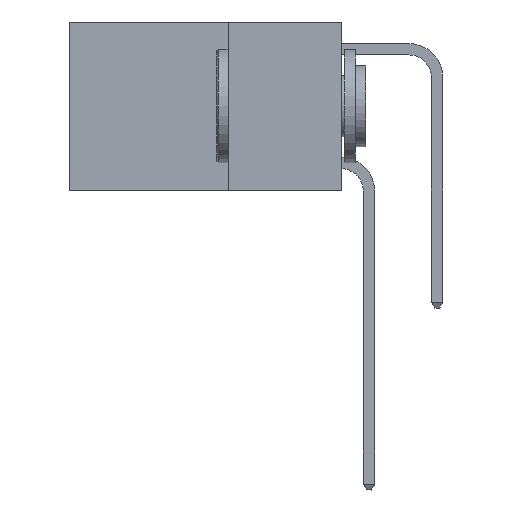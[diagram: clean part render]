
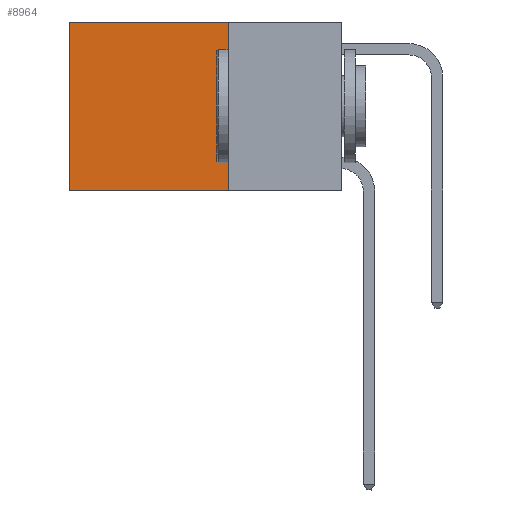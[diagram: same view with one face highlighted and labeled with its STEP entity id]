
A CAD part, left-side view. The second image highlights one B-rep face of the part: STEP entity #8964.
In plain terms, the highlighted planar face has unit normal (-1, 0, 0).
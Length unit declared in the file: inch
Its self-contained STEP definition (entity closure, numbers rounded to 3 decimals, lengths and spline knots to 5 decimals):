
#974 = VERTEX_POINT ( 'NONE', #7951 ) ;
#1046 = EDGE_CURVE ( 'NONE', #10269, #7973, #4621, .T. ) ;
#1064 = CARTESIAN_POINT ( 'NONE',  ( 0.2625, 0.25, 0. ) ) ;
#1311 = LINE ( 'NONE', #6498, #6515 ) ;
#1514 = PLANE ( 'NONE',  #8839 ) ;
#3802 = DIRECTION ( 'NONE',  ( 0., 0., -1. ) ) ;
#4322 = DIRECTION ( 'NONE',  ( 0., 1., 0. ) ) ;
#4621 = LINE ( 'NONE', #7030, #9663 ) ;
#5113 = EDGE_CURVE ( 'NONE', #6581, #974, #8562, .T. ) ;
#5207 = DIRECTION ( 'NONE',  ( 0., 0., -1. ) ) ;
#5236 = DIRECTION ( 'NONE',  ( 0., 1., 0. ) ) ;
#6070 = ORIENTED_EDGE ( 'NONE', *, *, #1046, .T. ) ;
#6247 = ORIENTED_EDGE ( 'NONE', *, *, #12987, .F. ) ;
#6341 = ORIENTED_EDGE ( 'NONE', *, *, #5113, .F. ) ;
#6498 = CARTESIAN_POINT ( 'NONE',  ( 0.2625, 0.25, 0. ) ) ;
#6515 = VECTOR ( 'NONE', #4322, 39.37008 ) ;
#6551 = ORIENTED_EDGE ( 'NONE', *, *, #10036, .T. ) ;
#6581 = VERTEX_POINT ( 'NONE', #1064 ) ;
#7030 = CARTESIAN_POINT ( 'NONE',  ( 0.2625, 0.6, 0. ) ) ;
#7479 = DIRECTION ( 'NONE',  ( 0., 0., -1. ) ) ;
#7480 = VECTOR ( 'NONE', #5236, 39.37008 ) ;
#7914 = CARTESIAN_POINT ( 'NONE',  ( 0.2625, 0.6, 0. ) ) ;
#7951 = CARTESIAN_POINT ( 'NONE',  ( 0.2625, 0.25, -0.37 ) ) ;
#7973 = VERTEX_POINT ( 'NONE', #11682 ) ;
#8378 = FACE_OUTER_BOUND ( 'NONE', #9348, .T. ) ;
#8562 = LINE ( 'NONE', #10663, #13103 ) ;
#8839 = AXIS2_PLACEMENT_3D ( 'NONE', #9188, #10248, #3802 ) ;
#8964 = ADVANCED_FACE ( 'NONE', ( #8378 ), #1514, .F. ) ;
#9188 = CARTESIAN_POINT ( 'NONE',  ( 0.2625, 0.25, 0. ) ) ;
#9348 = EDGE_LOOP ( 'NONE', ( #6070, #6247, #6341, #6551 ) ) ;
#9663 = VECTOR ( 'NONE', #5207, 39.37008 ) ;
#10036 = EDGE_CURVE ( 'NONE', #6581, #10269, #1311, .T. ) ;
#10248 = DIRECTION ( 'NONE',  ( 1., 0., 0. ) ) ;
#10269 = VERTEX_POINT ( 'NONE', #7914 ) ;
#10293 = LINE ( 'NONE', #12646, #7480 ) ;
#10663 = CARTESIAN_POINT ( 'NONE',  ( 0.2625, 0.25, 0. ) ) ;
#11682 = CARTESIAN_POINT ( 'NONE',  ( 0.2625, 0.6, -0.37 ) ) ;
#12646 = CARTESIAN_POINT ( 'NONE',  ( 0.2625, 0.25, -0.37 ) ) ;
#12987 = EDGE_CURVE ( 'NONE', #974, #7973, #10293, .T. ) ;
#13103 = VECTOR ( 'NONE', #7479, 39.37008 ) ;
